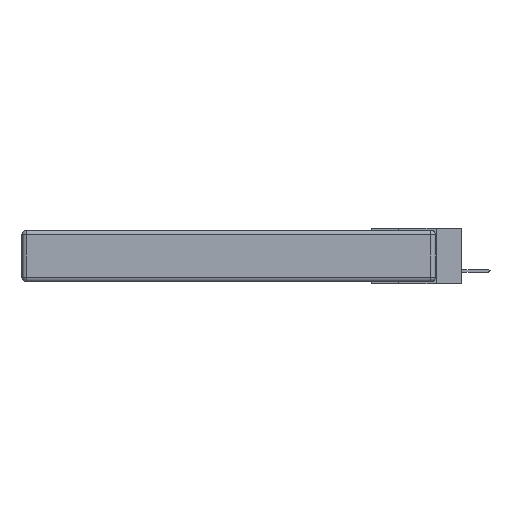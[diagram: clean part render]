
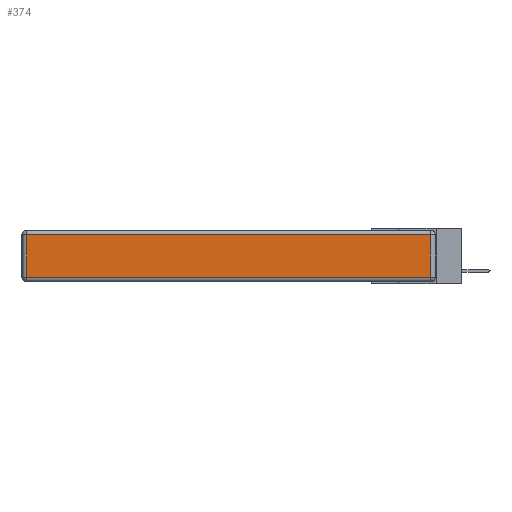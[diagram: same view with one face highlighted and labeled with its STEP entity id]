
A CAD part, left-side view. The second image highlights one B-rep face of the part: STEP entity #374.
In plain terms, the highlighted planar face has unit normal (-1, 0, 0).
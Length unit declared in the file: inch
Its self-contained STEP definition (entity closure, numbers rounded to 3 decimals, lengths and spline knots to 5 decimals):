
#210 = VERTEX_POINT ( 'NONE', #19275 ) ;
#374 = ADVANCED_FACE ( 'NONE', ( #17557 ), #20388, .T. ) ;
#411 = CARTESIAN_POINT ( 'NONE',  ( 0., 0.03, -0.03 ) ) ;
#2644 = ORIENTED_EDGE ( 'NONE', *, *, #5648, .T. ) ;
#4279 = CARTESIAN_POINT ( 'NONE',  ( 0., 2.72, -0.343 ) ) ;
#4522 = VECTOR ( 'NONE', #22424, 39.37008 ) ;
#4734 = CARTESIAN_POINT ( 'NONE',  ( 0., 2.75, -0.03 ) ) ;
#5648 = EDGE_CURVE ( 'NONE', #23302, #20174, #8741, .T. ) ;
#6482 = VECTOR ( 'NONE', #7072, 39.37008 ) ;
#7072 = DIRECTION ( 'NONE',  ( 0., 1., 0. ) ) ;
#7120 = EDGE_CURVE ( 'NONE', #26335, #210, #9288, .T. ) ;
#7127 = DIRECTION ( 'NONE',  ( 0., -1., 0. ) ) ;
#8741 = LINE ( 'NONE', #24836, #17503 ) ;
#9288 = LINE ( 'NONE', #4734, #6482 ) ;
#12076 = EDGE_CURVE ( 'NONE', #20174, #26335, #30005, .T. ) ;
#13058 = DIRECTION ( 'NONE',  ( 0., 0., 1. ) ) ;
#13477 = EDGE_CURVE ( 'NONE', #210, #23302, #20135, .T. ) ;
#15223 = CARTESIAN_POINT ( 'NONE',  ( 0., 0.03, -0.343 ) ) ;
#17503 = VECTOR ( 'NONE', #7127, 39.37008 ) ;
#17557 = FACE_OUTER_BOUND ( 'NONE', #31141, .T. ) ;
#17630 = DIRECTION ( 'NONE',  ( -1., 0., 0. ) ) ;
#18847 = ORIENTED_EDGE ( 'NONE', *, *, #12076, .T. ) ;
#19275 = CARTESIAN_POINT ( 'NONE',  ( 0., 2.72, -0.03 ) ) ;
#19625 = CARTESIAN_POINT ( 'NONE',  ( 0., 2.72, -0.313 ) ) ;
#20135 = LINE ( 'NONE', #4279, #26122 ) ;
#20174 = VERTEX_POINT ( 'NONE', #26236 ) ;
#20388 = PLANE ( 'NONE',  #26099 ) ;
#22424 = DIRECTION ( 'NONE',  ( 0., 0., 1. ) ) ;
#22733 = CARTESIAN_POINT ( 'NONE',  ( 0., 0., -0.343 ) ) ;
#23302 = VERTEX_POINT ( 'NONE', #19625 ) ;
#24836 = CARTESIAN_POINT ( 'NONE',  ( 0., 0., -0.313 ) ) ;
#26099 = AXIS2_PLACEMENT_3D ( 'NONE', #22733, #17630, #13058 ) ;
#26122 = VECTOR ( 'NONE', #31863, 39.37008 ) ;
#26236 = CARTESIAN_POINT ( 'NONE',  ( 0., 0.03, -0.313 ) ) ;
#26335 = VERTEX_POINT ( 'NONE', #411 ) ;
#27438 = ORIENTED_EDGE ( 'NONE', *, *, #7120, .T. ) ;
#30005 = LINE ( 'NONE', #15223, #4522 ) ;
#30931 = ORIENTED_EDGE ( 'NONE', *, *, #13477, .T. ) ;
#31141 = EDGE_LOOP ( 'NONE', ( #2644, #18847, #27438, #30931 ) ) ;
#31863 = DIRECTION ( 'NONE',  ( 0., 0., -1. ) ) ;
